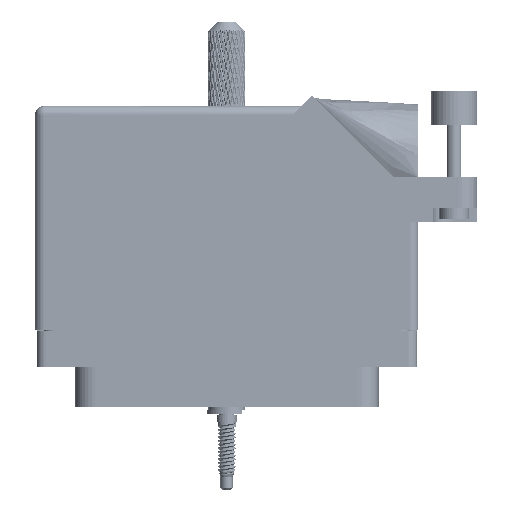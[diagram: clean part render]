
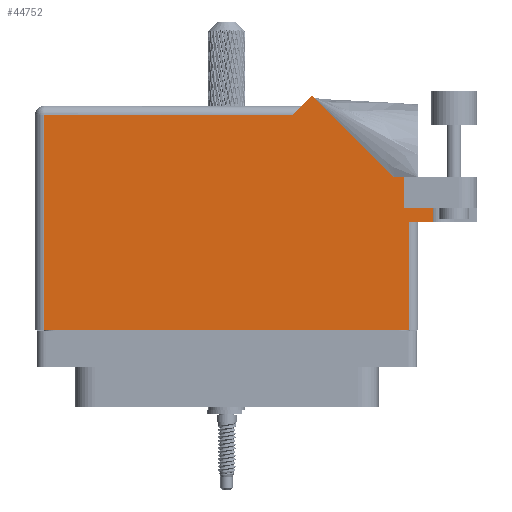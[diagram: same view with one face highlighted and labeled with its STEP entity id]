
A CAD part, front view. The second image highlights one B-rep face of the part: STEP entity #44752.
In plain terms, the highlighted face is planar.
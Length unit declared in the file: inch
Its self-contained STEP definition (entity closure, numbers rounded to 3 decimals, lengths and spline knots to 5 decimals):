
#515 = CARTESIAN_POINT ( 'NONE',  ( 1.206, 0.944, 0.455 ) ) ;
#2328 = VERTEX_POINT ( 'NONE', #28711 ) ;
#7397 = DIRECTION ( 'NONE',  ( -0.707, 0.707, 0. ) ) ;
#8173 = DIRECTION ( 'NONE',  ( 1., 0., 0. ) ) ;
#10059 = DIRECTION ( 'NONE',  ( 0., -1., 0. ) ) ;
#10463 = EDGE_CURVE ( 'NONE', #109706, #2328, #116354, .T. ) ;
#10845 = DIRECTION ( 'NONE',  ( -1., 0., 0. ) ) ;
#13095 = VECTOR ( 'NONE', #78645, 39.37008 ) ;
#13608 = CARTESIAN_POINT ( 'NONE',  ( 1.206, 0.731, 0.455 ) ) ;
#13833 = CARTESIAN_POINT ( 'NONE',  ( 1.206, 0.731, 0.455 ) ) ;
#15128 = CARTESIAN_POINT ( 'NONE',  ( -1.306, -0.1, 0.455 ) ) ;
#19945 = ORIENTED_EDGE ( 'NONE', *, *, #52686, .T. ) ;
#19978 = ORIENTED_EDGE ( 'NONE', *, *, #36491, .F. ) ;
#20258 = CARTESIAN_POINT ( 'NONE',  ( -1.306, 1.368, 0.455 ) ) ;
#20292 = VECTOR ( 'NONE', #58464, 39.37008 ) ;
#21993 = ORIENTED_EDGE ( 'NONE', *, *, #66940, .T. ) ;
#22022 = VECTOR ( 'NONE', #76452, 39.37008 ) ;
#23466 = DIRECTION ( 'NONE',  ( 1., 0., 0. ) ) ;
#24893 = CARTESIAN_POINT ( 'NONE',  ( 1.306, 0.637, 0.455 ) ) ;
#26486 = LINE ( 'NONE', #15128, #102095 ) ;
#28711 = CARTESIAN_POINT ( 'NONE',  ( 1.4075, 0.637, 0.455 ) ) ;
#29505 = VERTEX_POINT ( 'NONE', #76169 ) ;
#30945 = DIRECTION ( 'NONE',  ( -1., 0., 0. ) ) ;
#32009 = VERTEX_POINT ( 'NONE', #515 ) ;
#32256 = VECTOR ( 'NONE', #75826, 39.37008 ) ;
#34147 = CARTESIAN_POINT ( 'NONE',  ( 1.244, -0.1, 0.455 ) ) ;
#35188 = CARTESIAN_POINT ( 'NONE',  ( 1.14042, 0.944, 0.455 ) ) ;
#35485 = VERTEX_POINT ( 'NONE', #75569 ) ;
#36159 = LINE ( 'NONE', #86003, #22022 ) ;
#36491 = EDGE_CURVE ( 'NONE', #82382, #63673, #47708, .T. ) ;
#37589 = LINE ( 'NONE', #101290, #113194 ) ;
#38590 = VERTEX_POINT ( 'NONE', #115588 ) ;
#39426 = CARTESIAN_POINT ( 'NONE',  ( -1.306, 1.43, 0.455 ) ) ;
#43171 = LINE ( 'NONE', #20258, #88870 ) ;
#44752 = ADVANCED_FACE ( 'NONE', ( #86176 ), #94087, .F. ) ;
#45977 = DIRECTION ( 'NONE',  ( -1., 0., 0. ) ) ;
#47708 = LINE ( 'NONE', #13833, #87778 ) ;
#48552 = VECTOR ( 'NONE', #45977, 39.37008 ) ;
#50195 = CARTESIAN_POINT ( 'NONE',  ( 1.244, 0.637, 0.455 ) ) ;
#50685 = CARTESIAN_POINT ( 'NONE',  ( -1.244, -0.1, 0.455 ) ) ;
#52686 = EDGE_CURVE ( 'NONE', #104596, #106557, #26486, .T. ) ;
#54890 = EDGE_LOOP ( 'NONE', ( #19945, #90976, #100988, #116231, #19978, #90729, #86952, #71494, #93866, #84911, #21993 ) ) ;
#56343 = EDGE_CURVE ( 'NONE', #82382, #32009, #101587, .T. ) ;
#57724 = DIRECTION ( 'NONE',  ( 0., 0., -1. ) ) ;
#58464 = DIRECTION ( 'NONE',  ( 0., 1., 0. ) ) ;
#63673 = VERTEX_POINT ( 'NONE', #83783 ) ;
#66570 = CARTESIAN_POINT ( 'NONE',  ( 1.4075, 1.06177, 0.455 ) ) ;
#66940 = EDGE_CURVE ( 'NONE', #35485, #104596, #37589, .T. ) ;
#68847 = EDGE_CURVE ( 'NONE', #69825, #29505, #105798, .T. ) ;
#69234 = EDGE_CURVE ( 'NONE', #106557, #109706, #87209, .T. ) ;
#69825 = VERTEX_POINT ( 'NONE', #77169 ) ;
#71494 = ORIENTED_EDGE ( 'NONE', *, *, #68847, .T. ) ;
#73573 = VECTOR ( 'NONE', #8173, 39.37008 ) ;
#75569 = CARTESIAN_POINT ( 'NONE',  ( -1.244, 1.368, 0.455 ) ) ;
#75826 = DIRECTION ( 'NONE',  ( 0., -1., 0. ) ) ;
#76169 = CARTESIAN_POINT ( 'NONE',  ( 0.58371, 1.50071, 0.455 ) ) ;
#76452 = DIRECTION ( 'NONE',  ( -0.707, -0.707, 0. ) ) ;
#77169 = CARTESIAN_POINT ( 'NONE',  ( 1.14042, 0.944, 0.455 ) ) ;
#77614 = DIRECTION ( 'NONE',  ( 1., 0., 0. ) ) ;
#78231 = CARTESIAN_POINT ( 'NONE',  ( 1.244, 0.637, 0.455 ) ) ;
#78645 = DIRECTION ( 'NONE',  ( 0., 1., 0. ) ) ;
#80871 = LINE ( 'NONE', #66570, #32256 ) ;
#81627 = VECTOR ( 'NONE', #7397, 39.37008 ) ;
#82382 = VERTEX_POINT ( 'NONE', #13608 ) ;
#82790 = EDGE_CURVE ( 'NONE', #38590, #35485, #43171, .T. ) ;
#83783 = CARTESIAN_POINT ( 'NONE',  ( 1.4075, 0.731, 0.455 ) ) ;
#84911 = ORIENTED_EDGE ( 'NONE', *, *, #82790, .T. ) ;
#86003 = CARTESIAN_POINT ( 'NONE',  ( 0.513, 1.43, 0.455 ) ) ;
#86176 = FACE_OUTER_BOUND ( 'NONE', #54890, .T. ) ;
#86952 = ORIENTED_EDGE ( 'NONE', *, *, #111931, .T. ) ;
#87209 = LINE ( 'NONE', #78231, #13095 ) ;
#87778 = VECTOR ( 'NONE', #77614, 39.37008 ) ;
#88870 = VECTOR ( 'NONE', #30945, 39.37008 ) ;
#90729 = ORIENTED_EDGE ( 'NONE', *, *, #56343, .T. ) ;
#90976 = ORIENTED_EDGE ( 'NONE', *, *, #69234, .T. ) ;
#93866 = ORIENTED_EDGE ( 'NONE', *, *, #96085, .T. ) ;
#94087 = PLANE ( 'NONE',  #117930 ) ;
#96085 = EDGE_CURVE ( 'NONE', #29505, #38590, #36159, .T. ) ;
#97200 = LINE ( 'NONE', #107457, #48552 ) ;
#100988 = ORIENTED_EDGE ( 'NONE', *, *, #10463, .T. ) ;
#101290 = CARTESIAN_POINT ( 'NONE',  ( -1.244, -0.1, 0.455 ) ) ;
#101587 = LINE ( 'NONE', #103582, #20292 ) ;
#102095 = VECTOR ( 'NONE', #23466, 39.37008 ) ;
#103582 = CARTESIAN_POINT ( 'NONE',  ( 1.206, 0.731, 0.455 ) ) ;
#104596 = VERTEX_POINT ( 'NONE', #50685 ) ;
#105798 = LINE ( 'NONE', #35188, #81627 ) ;
#106557 = VERTEX_POINT ( 'NONE', #34147 ) ;
#107457 = CARTESIAN_POINT ( 'NONE',  ( 1.706, 0.944, 0.455 ) ) ;
#109706 = VERTEX_POINT ( 'NONE', #50195 ) ;
#111931 = EDGE_CURVE ( 'NONE', #32009, #69825, #97200, .T. ) ;
#113194 = VECTOR ( 'NONE', #10059, 39.37008 ) ;
#115493 = EDGE_CURVE ( 'NONE', #63673, #2328, #80871, .T. ) ;
#115588 = CARTESIAN_POINT ( 'NONE',  ( 0.451, 1.368, 0.455 ) ) ;
#116231 = ORIENTED_EDGE ( 'NONE', *, *, #115493, .F. ) ;
#116354 = LINE ( 'NONE', #24893, #73573 ) ;
#117930 = AXIS2_PLACEMENT_3D ( 'NONE', #39426, #57724, #10845 ) ;
